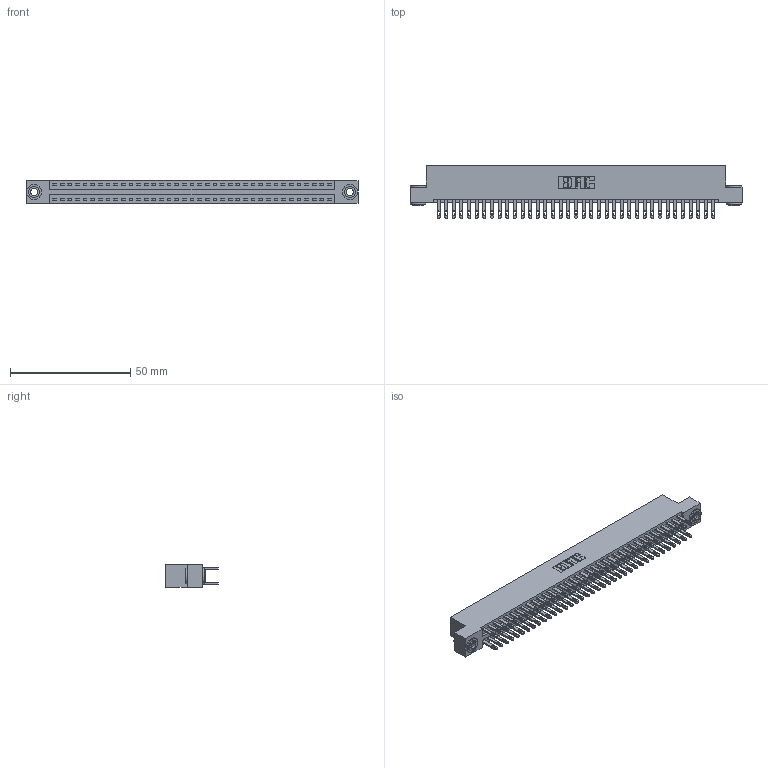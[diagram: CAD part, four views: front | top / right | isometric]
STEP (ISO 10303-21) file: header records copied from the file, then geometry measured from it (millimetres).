
FILE_DESCRIPTION (( 'STEP AP203' ), '1' );
FILE_NAME ('896-074-500-203.STEP', '2021-07-28T01:30:48', ( '' ), ( '' ), 'SwSTEP 2.0', 'SolidWorks 2020', '' );
FILE_SCHEMA (( 'CONFIG_CONTROL_DESIGN' ));
Length unit declared in the file: inch
Products named in the file (4): 846 Part_Flush Mounting Lugs - 0.156 Dia-TH; 345-292-001_345-293-100; 345-250-002_345-250-002-102; 896-074-500-203
Assembly tree (77 placements, depth 2):
  896-074-500-203
    846 Part_Flush Mounting Lugs - 0.156 Dia-TH
    345-292-001_345-293-100  x74
    345-250-002_345-250-002-102  x2
Bounding box: 138.05 x 21.84 x 9.4 mm (x, y, z)
Volume: 13668.2 mm3; surface area: 19697.9 mm2
Topology: 77 solids, 77 shells, 3712 faces, 11283 edges, 7518 vertices
Faces by surface type: plane 2232, cylinder 1472, cone 8
Entity records: 25400 total; most frequent: CARTESIAN_POINT 4167, ORIENTED_EDGE 4094, DIRECTION 3757, EDGE_CURVE 2047, VECTOR 1739, LINE 1739, VERTEX_POINT 1362, AXIS2_PLACEMENT_3D 1009
